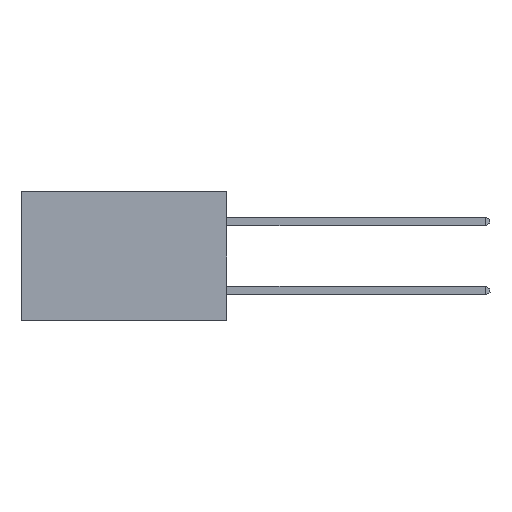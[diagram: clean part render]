
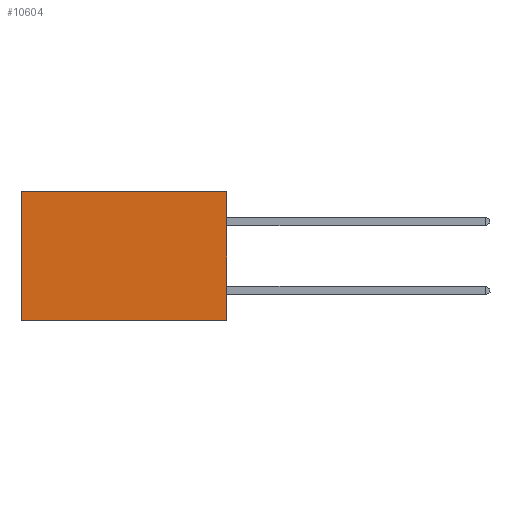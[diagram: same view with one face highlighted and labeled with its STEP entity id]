
A CAD part, left-side view. The second image highlights one B-rep face of the part: STEP entity #10604.
In plain terms, the highlighted planar face has unit normal (-1, 0, 0).
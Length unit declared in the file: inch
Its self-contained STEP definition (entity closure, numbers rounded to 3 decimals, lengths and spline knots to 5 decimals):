
#498 = CARTESIAN_POINT ( 'NONE',  ( 0.277, 0., -0.37 ) ) ;
#607 = DIRECTION ( 'NONE',  ( 0., 0., -1. ) ) ;
#983 = DIRECTION ( 'NONE',  ( 0., 0., -1. ) ) ;
#1792 = CARTESIAN_POINT ( 'NONE',  ( 0.277, 0., 0. ) ) ;
#2068 = FACE_OUTER_BOUND ( 'NONE', #2223, .T. ) ;
#2223 = EDGE_LOOP ( 'NONE', ( #8885, #3416, #9459, #11226 ) ) ;
#2564 = LINE ( 'NONE', #10313, #10529 ) ;
#2949 = CARTESIAN_POINT ( 'NONE',  ( 0.277, 0.59, -0.37 ) ) ;
#3009 = LINE ( 'NONE', #19379, #10976 ) ;
#3416 = ORIENTED_EDGE ( 'NONE', *, *, #15261, .F. ) ;
#5553 = VERTEX_POINT ( 'NONE', #13307 ) ;
#7183 = CARTESIAN_POINT ( 'NONE',  ( 0.277, 0., 0. ) ) ;
#8126 = EDGE_CURVE ( 'NONE', #5553, #8477, #2564, .T. ) ;
#8477 = VERTEX_POINT ( 'NONE', #2949 ) ;
#8885 = ORIENTED_EDGE ( 'NONE', *, *, #8126, .T. ) ;
#9459 = ORIENTED_EDGE ( 'NONE', *, *, #16032, .F. ) ;
#9492 = VERTEX_POINT ( 'NONE', #18866 ) ;
#9950 = DIRECTION ( 'NONE',  ( 0., 0., -1. ) ) ;
#9952 = AXIS2_PLACEMENT_3D ( 'NONE', #19768, #10505, #983 ) ;
#10313 = CARTESIAN_POINT ( 'NONE',  ( 0.277, 0.59, -0.37 ) ) ;
#10505 = DIRECTION ( 'NONE',  ( 1., 0., 0. ) ) ;
#10529 = VECTOR ( 'NONE', #9950, 39.37008 ) ;
#10541 = EDGE_CURVE ( 'NONE', #15164, #5553, #19722, .T. ) ;
#10604 = ADVANCED_FACE ( 'NONE', ( #2068 ), #13605, .F. ) ;
#10976 = VECTOR ( 'NONE', #607, 39.37008 ) ;
#11226 = ORIENTED_EDGE ( 'NONE', *, *, #10541, .T. ) ;
#11805 = LINE ( 'NONE', #498, #16022 ) ;
#13172 = DIRECTION ( 'NONE',  ( 0., 1., 0. ) ) ;
#13307 = CARTESIAN_POINT ( 'NONE',  ( 0.277, 0.59, 0. ) ) ;
#13605 = PLANE ( 'NONE',  #9952 ) ;
#15164 = VERTEX_POINT ( 'NONE', #1792 ) ;
#15261 = EDGE_CURVE ( 'NONE', #9492, #8477, #11805, .T. ) ;
#16022 = VECTOR ( 'NONE', #13172, 39.37008 ) ;
#16032 = EDGE_CURVE ( 'NONE', #15164, #9492, #3009, .T. ) ;
#18866 = CARTESIAN_POINT ( 'NONE',  ( 0.277, 0., -0.37 ) ) ;
#19379 = CARTESIAN_POINT ( 'NONE',  ( 0.277, 0., -0.37 ) ) ;
#19629 = DIRECTION ( 'NONE',  ( 0., 1., 0. ) ) ;
#19722 = LINE ( 'NONE', #7183, #20185 ) ;
#19768 = CARTESIAN_POINT ( 'NONE',  ( 0.277, 0., -0.37 ) ) ;
#20185 = VECTOR ( 'NONE', #19629, 39.37008 ) ;
